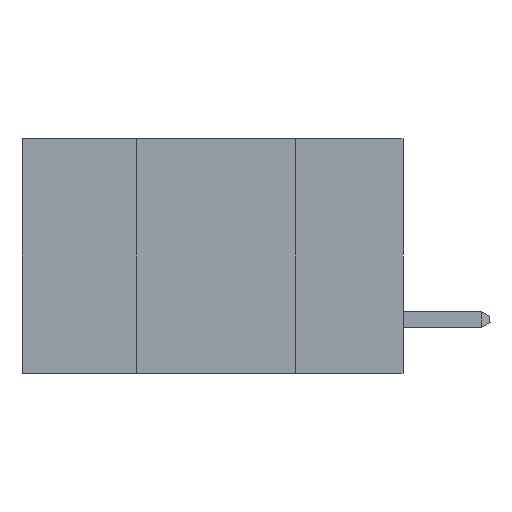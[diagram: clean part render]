
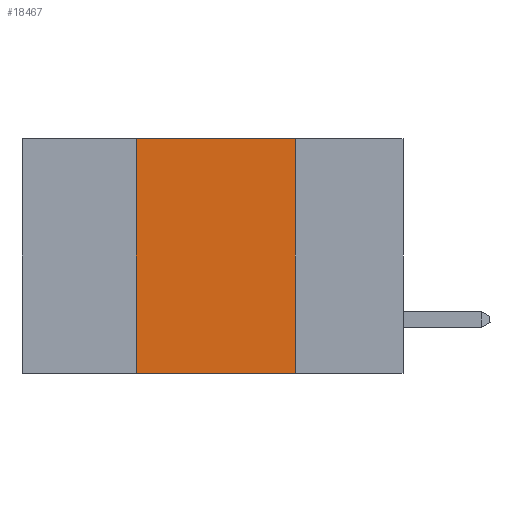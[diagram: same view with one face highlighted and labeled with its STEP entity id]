
A CAD part, left-side view. The second image highlights one B-rep face of the part: STEP entity #18467.
In plain terms, the highlighted planar face has unit normal (-1, 0, 0).
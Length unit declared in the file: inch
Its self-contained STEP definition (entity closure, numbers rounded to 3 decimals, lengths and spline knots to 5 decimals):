
#460 = LINE ( 'NONE', #20466, #31931 ) ;
#727 = VECTOR ( 'NONE', #6675, 39.37008 ) ;
#1069 = CARTESIAN_POINT ( 'NONE',  ( 0., 0.17, -0.37 ) ) ;
#1196 = LINE ( 'NONE', #1298, #28273 ) ;
#1257 = CARTESIAN_POINT ( 'NONE',  ( 0., 0.6, -0.37 ) ) ;
#1298 = CARTESIAN_POINT ( 'NONE',  ( 0., 0.6, 0. ) ) ;
#2516 = VERTEX_POINT ( 'NONE', #16692 ) ;
#5274 = DIRECTION ( 'NONE',  ( 0., 0., 1. ) ) ;
#6193 = EDGE_LOOP ( 'NONE', ( #27012, #13192, #9912, #18022 ) ) ;
#6463 = CARTESIAN_POINT ( 'NONE',  ( 0., 0.6, 0. ) ) ;
#6675 = DIRECTION ( 'NONE',  ( 0., -1., 0. ) ) ;
#9039 = DIRECTION ( 'NONE',  ( 1., 0., 0. ) ) ;
#9529 = CARTESIAN_POINT ( 'NONE',  ( 0., 0.42, 0. ) ) ;
#9912 = ORIENTED_EDGE ( 'NONE', *, *, #28883, .F. ) ;
#10289 = EDGE_CURVE ( 'NONE', #2516, #30333, #460, .T. ) ;
#12184 = EDGE_CURVE ( 'NONE', #14622, #30333, #28985, .T. ) ;
#12239 = LINE ( 'NONE', #25789, #24231 ) ;
#13192 = ORIENTED_EDGE ( 'NONE', *, *, #32898, .F. ) ;
#13851 = CARTESIAN_POINT ( 'NONE',  ( 0., 0.42, -0.37 ) ) ;
#14251 = DIRECTION ( 'NONE',  ( 0., 0., -1. ) ) ;
#14356 = PLANE ( 'NONE',  #24489 ) ;
#14622 = VERTEX_POINT ( 'NONE', #13851 ) ;
#16692 = CARTESIAN_POINT ( 'NONE',  ( 0., 0.17, 0. ) ) ;
#18022 = ORIENTED_EDGE ( 'NONE', *, *, #12184, .T. ) ;
#18467 = ADVANCED_FACE ( 'NONE', ( #20555 ), #14356, .F. ) ;
#20466 = CARTESIAN_POINT ( 'NONE',  ( 0., 0.17, 0. ) ) ;
#20555 = FACE_OUTER_BOUND ( 'NONE', #6193, .T. ) ;
#24231 = VECTOR ( 'NONE', #5274, 39.37008 ) ;
#24489 = AXIS2_PLACEMENT_3D ( 'NONE', #6463, #9039, #14251 ) ;
#25789 = CARTESIAN_POINT ( 'NONE',  ( 0., 0.42, 0. ) ) ;
#26820 = VERTEX_POINT ( 'NONE', #9529 ) ;
#27012 = ORIENTED_EDGE ( 'NONE', *, *, #10289, .F. ) ;
#28273 = VECTOR ( 'NONE', #29457, 39.37008 ) ;
#28883 = EDGE_CURVE ( 'NONE', #14622, #26820, #12239, .T. ) ;
#28985 = LINE ( 'NONE', #1257, #727 ) ;
#29457 = DIRECTION ( 'NONE',  ( 0., -1., 0. ) ) ;
#30333 = VERTEX_POINT ( 'NONE', #1069 ) ;
#30499 = DIRECTION ( 'NONE',  ( 0., 0., -1. ) ) ;
#31931 = VECTOR ( 'NONE', #30499, 39.37008 ) ;
#32898 = EDGE_CURVE ( 'NONE', #26820, #2516, #1196, .T. ) ;
